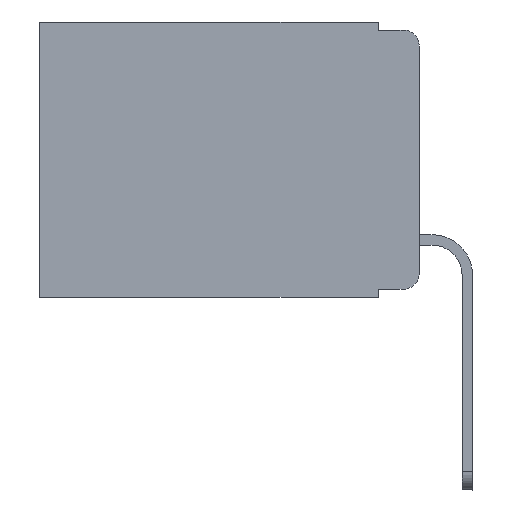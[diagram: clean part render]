
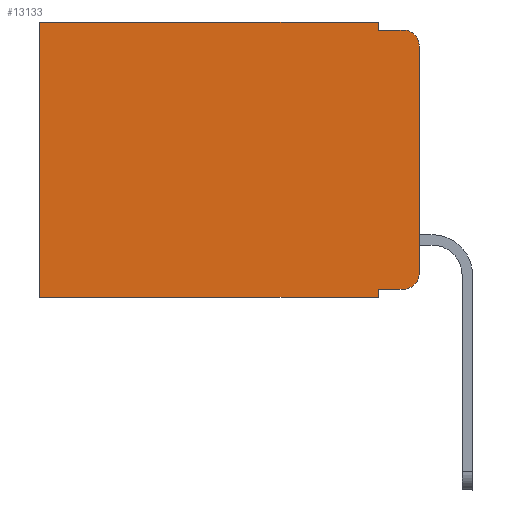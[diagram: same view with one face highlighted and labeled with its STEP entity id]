
A CAD part, left-side view. The second image highlights one B-rep face of the part: STEP entity #13133.
In plain terms, the highlighted planar face has unit normal (-1, 0, 0).
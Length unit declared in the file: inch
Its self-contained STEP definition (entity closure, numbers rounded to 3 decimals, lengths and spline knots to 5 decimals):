
#151 = DIRECTION ( 'NONE',  ( -1., 0., 0. ) ) ;
#436 = DIRECTION ( 'NONE',  ( 0., 1., 0. ) ) ;
#702 = LINE ( 'NONE', #6674, #16448 ) ;
#734 = AXIS2_PLACEMENT_3D ( 'NONE', #4577, #2460, #18651 ) ;
#746 = CARTESIAN_POINT ( 'NONE',  ( 0.298, 0.051, 0. ) ) ;
#1153 = VERTEX_POINT ( 'NONE', #14825 ) ;
#1297 = EDGE_CURVE ( 'NONE', #5505, #19749, #6889, .T. ) ;
#1529 = CARTESIAN_POINT ( 'NONE',  ( 0.298, 0.473, -0.343 ) ) ;
#1571 = EDGE_CURVE ( 'NONE', #1153, #10025, #18451, .T. ) ;
#2324 = LINE ( 'NONE', #5859, #5036 ) ;
#2394 = VERTEX_POINT ( 'NONE', #3834 ) ;
#2460 = DIRECTION ( 'NONE',  ( 1., 0., 0. ) ) ;
#3384 = CARTESIAN_POINT ( 'NONE',  ( 0.298, 0.02, -0.01 ) ) ;
#3395 = VECTOR ( 'NONE', #18350, 39.37008 ) ;
#3399 = VERTEX_POINT ( 'NONE', #1529 ) ;
#3691 = CARTESIAN_POINT ( 'NONE',  ( 0.298, 0.051, -0.01 ) ) ;
#3834 = CARTESIAN_POINT ( 'NONE',  ( 0.298, 0.051, -0.343 ) ) ;
#3925 = LINE ( 'NONE', #19887, #12895 ) ;
#4110 = EDGE_CURVE ( 'NONE', #8872, #2394, #11609, .T. ) ;
#4203 = EDGE_CURVE ( 'NONE', #8872, #21001, #5337, .T. ) ;
#4379 = DIRECTION ( 'NONE',  ( 0., 0., -1. ) ) ;
#4577 = CARTESIAN_POINT ( 'NONE',  ( 0.298, 0., 0. ) ) ;
#5036 = VECTOR ( 'NONE', #436, 39.37008 ) ;
#5337 = LINE ( 'NONE', #19391, #11286 ) ;
#5369 = ORIENTED_EDGE ( 'NONE', *, *, #4110, .F. ) ;
#5505 = VERTEX_POINT ( 'NONE', #3691 ) ;
#5583 = EDGE_CURVE ( 'NONE', #6893, #5505, #3925, .T. ) ;
#5859 = CARTESIAN_POINT ( 'NONE',  ( 0.298, 0., 0. ) ) ;
#5933 = DIRECTION ( 'NONE',  ( 0., 0., -1. ) ) ;
#6674 = CARTESIAN_POINT ( 'NONE',  ( 0.298, 0., -0.343 ) ) ;
#6889 = LINE ( 'NONE', #15526, #12849 ) ;
#6893 = VERTEX_POINT ( 'NONE', #10472 ) ;
#7068 = EDGE_CURVE ( 'NONE', #6893, #22360, #2324, .T. ) ;
#7130 = VECTOR ( 'NONE', #9955, 39.37008 ) ;
#7295 = ORIENTED_EDGE ( 'NONE', *, *, #1297, .F. ) ;
#7345 = DIRECTION ( 'NONE',  ( 0., 0., -1. ) ) ;
#7818 = CARTESIAN_POINT ( 'NONE',  ( 0.298, 0., 0. ) ) ;
#7862 = CARTESIAN_POINT ( 'NONE',  ( 0.298, 0., -0.313 ) ) ;
#8518 = DIRECTION ( 'NONE',  ( 0., -1., 0. ) ) ;
#8797 = CARTESIAN_POINT ( 'NONE',  ( 0.298, 0.473, 0. ) ) ;
#8872 = VERTEX_POINT ( 'NONE', #11509 ) ;
#9003 = DIRECTION ( 'NONE',  ( -1., 0., 0. ) ) ;
#9805 = CIRCLE ( 'NONE', #23009, 0.02 ) ;
#9955 = DIRECTION ( 'NONE',  ( 0., 0., -1. ) ) ;
#10025 = VERTEX_POINT ( 'NONE', #7862 ) ;
#10102 = VECTOR ( 'NONE', #4379, 39.37008 ) ;
#10472 = CARTESIAN_POINT ( 'NONE',  ( 0.298, 0.051, 0. ) ) ;
#10785 = EDGE_CURVE ( 'NONE', #21001, #10025, #9805, .T. ) ;
#11137 = DIRECTION ( 'NONE',  ( 0., 0., -1. ) ) ;
#11286 = VECTOR ( 'NONE', #8518, 39.37008 ) ;
#11509 = CARTESIAN_POINT ( 'NONE',  ( 0.298, 0.051, -0.333 ) ) ;
#11571 = AXIS2_PLACEMENT_3D ( 'NONE', #19876, #151, #7345 ) ;
#11609 = LINE ( 'NONE', #746, #7130 ) ;
#12068 = ORIENTED_EDGE ( 'NONE', *, *, #10785, .T. ) ;
#12849 = VECTOR ( 'NONE', #15635, 39.37008 ) ;
#12895 = VECTOR ( 'NONE', #11137, 39.37008 ) ;
#12912 = CARTESIAN_POINT ( 'NONE',  ( 0.298, 0.02, -0.313 ) ) ;
#13133 = ADVANCED_FACE ( 'NONE', ( #16760 ), #20769, .F. ) ;
#14825 = CARTESIAN_POINT ( 'NONE',  ( 0.298, 0., -0.03 ) ) ;
#14926 = LINE ( 'NONE', #16580, #3395 ) ;
#14989 = DIRECTION ( 'NONE',  ( 0., 1., 0. ) ) ;
#15395 = ORIENTED_EDGE ( 'NONE', *, *, #16438, .T. ) ;
#15526 = CARTESIAN_POINT ( 'NONE',  ( 0.298, 0.051, -0.01 ) ) ;
#15635 = DIRECTION ( 'NONE',  ( 0., -1., 0. ) ) ;
#15850 = EDGE_CURVE ( 'NONE', #2394, #3399, #702, .T. ) ;
#16438 = EDGE_CURVE ( 'NONE', #1153, #19749, #23273, .T. ) ;
#16448 = VECTOR ( 'NONE', #14989, 39.37008 ) ;
#16580 = CARTESIAN_POINT ( 'NONE',  ( 0.298, 0.473, 0. ) ) ;
#16760 = FACE_OUTER_BOUND ( 'NONE', #21987, .T. ) ;
#16805 = ORIENTED_EDGE ( 'NONE', *, *, #20330, .T. ) ;
#18350 = DIRECTION ( 'NONE',  ( 0., 0., -1. ) ) ;
#18451 = LINE ( 'NONE', #7818, #10102 ) ;
#18651 = DIRECTION ( 'NONE',  ( 0., 0., -1. ) ) ;
#19209 = ORIENTED_EDGE ( 'NONE', *, *, #5583, .F. ) ;
#19257 = CARTESIAN_POINT ( 'NONE',  ( 0.298, 0.02, -0.333 ) ) ;
#19391 = CARTESIAN_POINT ( 'NONE',  ( 0.298, 0.051, -0.333 ) ) ;
#19749 = VERTEX_POINT ( 'NONE', #3384 ) ;
#19876 = CARTESIAN_POINT ( 'NONE',  ( 0.298, 0.02, -0.03 ) ) ;
#19887 = CARTESIAN_POINT ( 'NONE',  ( 0.298, 0.051, 0. ) ) ;
#19987 = ORIENTED_EDGE ( 'NONE', *, *, #4203, .T. ) ;
#20001 = ORIENTED_EDGE ( 'NONE', *, *, #15850, .F. ) ;
#20330 = EDGE_CURVE ( 'NONE', #22360, #3399, #14926, .T. ) ;
#20739 = ORIENTED_EDGE ( 'NONE', *, *, #1571, .F. ) ;
#20769 = PLANE ( 'NONE',  #734 ) ;
#21001 = VERTEX_POINT ( 'NONE', #19257 ) ;
#21594 = ORIENTED_EDGE ( 'NONE', *, *, #7068, .T. ) ;
#21987 = EDGE_LOOP ( 'NONE', ( #20739, #15395, #7295, #19209, #21594, #16805, #20001, #5369, #19987, #12068 ) ) ;
#22360 = VERTEX_POINT ( 'NONE', #8797 ) ;
#23009 = AXIS2_PLACEMENT_3D ( 'NONE', #12912, #9003, #5933 ) ;
#23273 = CIRCLE ( 'NONE', #11571, 0.02 ) ;
